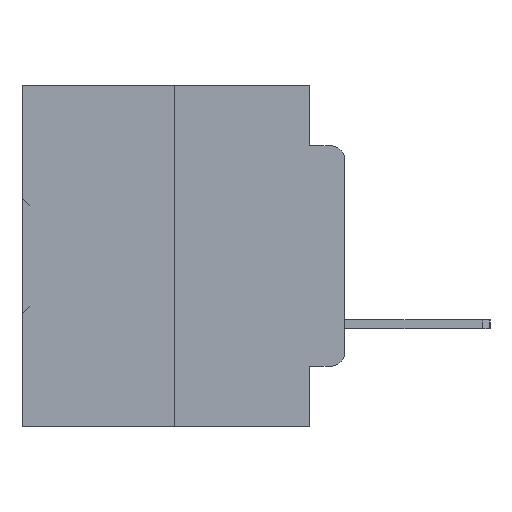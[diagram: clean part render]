
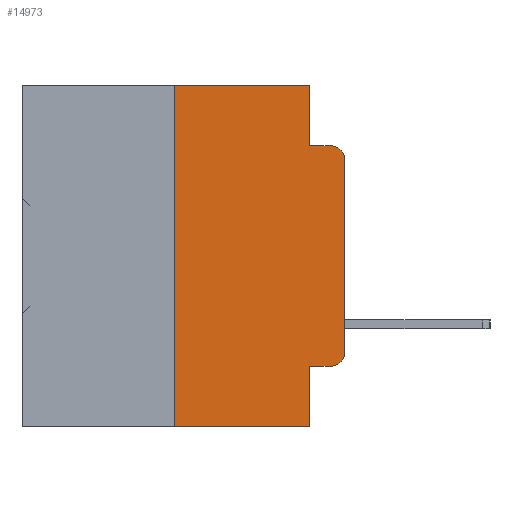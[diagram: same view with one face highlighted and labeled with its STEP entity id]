
A CAD part, left-side view. The second image highlights one B-rep face of the part: STEP entity #14973.
In plain terms, the highlighted planar face has unit normal (-1, 0, 0).
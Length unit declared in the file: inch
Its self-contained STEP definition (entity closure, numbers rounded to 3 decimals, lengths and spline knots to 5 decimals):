
#260 = CARTESIAN_POINT ( 'NONE',  ( 0., 0.25, -0.5 ) ) ;
#705 = VECTOR ( 'NONE', #7834, 39.37008 ) ;
#1303 = EDGE_CURVE ( 'NONE', #7194, #5282, #11119, .T. ) ;
#1907 = CARTESIAN_POINT ( 'NONE',  ( 0., 0.051, -0.4115 ) ) ;
#3157 = ORIENTED_EDGE ( 'NONE', *, *, #1303, .F. ) ;
#3260 = EDGE_CURVE ( 'NONE', #16669, #8296, #23354, .T. ) ;
#4362 = EDGE_CURVE ( 'NONE', #15178, #6514, #33932, .T. ) ;
#4369 = CARTESIAN_POINT ( 'NONE',  ( 0., 0., -0.1085 ) ) ;
#4507 = AXIS2_PLACEMENT_3D ( 'NONE', #18958, #19082, #15504 ) ;
#4655 = LINE ( 'NONE', #19867, #26301 ) ;
#4826 = PLANE ( 'NONE',  #6511 ) ;
#4999 = ORIENTED_EDGE ( 'NONE', *, *, #33340, .T. ) ;
#5282 = VERTEX_POINT ( 'NONE', #15598 ) ;
#5660 = CARTESIAN_POINT ( 'NONE',  ( 0., 0.02, -0.4115 ) ) ;
#5827 = CARTESIAN_POINT ( 'NONE',  ( 0., 0.051, -0.0885 ) ) ;
#5829 = ORIENTED_EDGE ( 'NONE', *, *, #6558, .T. ) ;
#6009 = VECTOR ( 'NONE', #35574, 39.37008 ) ;
#6118 = EDGE_CURVE ( 'NONE', #5282, #16669, #17180, .T. ) ;
#6511 = AXIS2_PLACEMENT_3D ( 'NONE', #24610, #27393, #10530 ) ;
#6514 = VERTEX_POINT ( 'NONE', #28648 ) ;
#6558 = EDGE_CURVE ( 'NONE', #7194, #25589, #17139, .T. ) ;
#7194 = VERTEX_POINT ( 'NONE', #260 ) ;
#7834 = DIRECTION ( 'NONE',  ( 0., 0., -1. ) ) ;
#8296 = VERTEX_POINT ( 'NONE', #5827 ) ;
#8911 = ORIENTED_EDGE ( 'NONE', *, *, #10861, .F. ) ;
#9947 = ORIENTED_EDGE ( 'NONE', *, *, #21044, .F. ) ;
#10082 = DIRECTION ( 'NONE',  ( 0., -1., 0. ) ) ;
#10233 = VECTOR ( 'NONE', #12822, 39.37008 ) ;
#10530 = DIRECTION ( 'NONE',  ( 0., 0., -1. ) ) ;
#10575 = VECTOR ( 'NONE', #10082, 39.37008 ) ;
#10861 = EDGE_CURVE ( 'NONE', #8296, #23716, #4655, .T. ) ;
#11119 = LINE ( 'NONE', #24066, #10233 ) ;
#11692 = DIRECTION ( 'NONE',  ( -1., 0., 0. ) ) ;
#11818 = CARTESIAN_POINT ( 'NONE',  ( 0., 0.02, -0.0885 ) ) ;
#12822 = DIRECTION ( 'NONE',  ( 0., 0., 1. ) ) ;
#14581 = AXIS2_PLACEMENT_3D ( 'NONE', #28563, #11692, #31351 ) ;
#14878 = DIRECTION ( 'NONE',  ( 0., -1., 0. ) ) ;
#14973 = ADVANCED_FACE ( 'NONE', ( #31675 ), #4826, .F. ) ;
#15167 = CARTESIAN_POINT ( 'NONE',  ( 0., 0.051, -0.5 ) ) ;
#15178 = VERTEX_POINT ( 'NONE', #5660 ) ;
#15310 = LINE ( 'NONE', #34096, #29376 ) ;
#15504 = DIRECTION ( 'NONE',  ( 0., 0., -1. ) ) ;
#15598 = CARTESIAN_POINT ( 'NONE',  ( 0., 0.25, 0. ) ) ;
#16669 = VERTEX_POINT ( 'NONE', #34894 ) ;
#16941 = EDGE_LOOP ( 'NONE', ( #32120, #31257, #8911, #18988, #31391, #3157, #5829, #9947, #4999, #34046 ) ) ;
#17139 = LINE ( 'NONE', #31668, #32063 ) ;
#17180 = LINE ( 'NONE', #21353, #10575 ) ;
#17357 = DIRECTION ( 'NONE',  ( 0., 0., 1. ) ) ;
#17743 = VERTEX_POINT ( 'NONE', #4369 ) ;
#18958 = CARTESIAN_POINT ( 'NONE',  ( 0., 0.02, -0.3915 ) ) ;
#18988 = ORIENTED_EDGE ( 'NONE', *, *, #3260, .F. ) ;
#19082 = DIRECTION ( 'NONE',  ( -1., 0., 0. ) ) ;
#19867 = CARTESIAN_POINT ( 'NONE',  ( 0., 0.051, -0.0885 ) ) ;
#21044 = EDGE_CURVE ( 'NONE', #23569, #25589, #23047, .T. ) ;
#21353 = CARTESIAN_POINT ( 'NONE',  ( 0., 0.473, 0. ) ) ;
#21973 = LINE ( 'NONE', #1907, #6009 ) ;
#22466 = CARTESIAN_POINT ( 'NONE',  ( 0., 0.051, -0.4115 ) ) ;
#22725 = DIRECTION ( 'NONE',  ( 0., -1., 0. ) ) ;
#23047 = LINE ( 'NONE', #27847, #29594 ) ;
#23354 = LINE ( 'NONE', #34065, #705 ) ;
#23569 = VERTEX_POINT ( 'NONE', #22466 ) ;
#23716 = VERTEX_POINT ( 'NONE', #11818 ) ;
#24066 = CARTESIAN_POINT ( 'NONE',  ( 0., 0.25, 0. ) ) ;
#24610 = CARTESIAN_POINT ( 'NONE',  ( 0., 0.473, 0. ) ) ;
#25589 = VERTEX_POINT ( 'NONE', #15167 ) ;
#25976 = EDGE_CURVE ( 'NONE', #17743, #23716, #35539, .T. ) ;
#26301 = VECTOR ( 'NONE', #22725, 39.37008 ) ;
#27393 = DIRECTION ( 'NONE',  ( 1., 0., 0. ) ) ;
#27829 = EDGE_CURVE ( 'NONE', #6514, #17743, #15310, .T. ) ;
#27847 = CARTESIAN_POINT ( 'NONE',  ( 0., 0.051, 0. ) ) ;
#28563 = CARTESIAN_POINT ( 'NONE',  ( 0., 0.02, -0.1085 ) ) ;
#28648 = CARTESIAN_POINT ( 'NONE',  ( 0., 0., -0.3915 ) ) ;
#29376 = VECTOR ( 'NONE', #17357, 39.37008 ) ;
#29594 = VECTOR ( 'NONE', #36286, 39.37008 ) ;
#31257 = ORIENTED_EDGE ( 'NONE', *, *, #25976, .T. ) ;
#31351 = DIRECTION ( 'NONE',  ( 0., 0., -1. ) ) ;
#31391 = ORIENTED_EDGE ( 'NONE', *, *, #6118, .F. ) ;
#31668 = CARTESIAN_POINT ( 'NONE',  ( 0., 0.473, -0.5 ) ) ;
#31675 = FACE_OUTER_BOUND ( 'NONE', #16941, .T. ) ;
#32063 = VECTOR ( 'NONE', #14878, 39.37008 ) ;
#32120 = ORIENTED_EDGE ( 'NONE', *, *, #27829, .T. ) ;
#33340 = EDGE_CURVE ( 'NONE', #23569, #15178, #21973, .T. ) ;
#33932 = CIRCLE ( 'NONE', #4507, 0.02 ) ;
#34046 = ORIENTED_EDGE ( 'NONE', *, *, #4362, .T. ) ;
#34065 = CARTESIAN_POINT ( 'NONE',  ( 0., 0.051, 0. ) ) ;
#34096 = CARTESIAN_POINT ( 'NONE',  ( 0., 0., 0. ) ) ;
#34894 = CARTESIAN_POINT ( 'NONE',  ( 0., 0.051, 0. ) ) ;
#35539 = CIRCLE ( 'NONE', #14581, 0.02 ) ;
#35574 = DIRECTION ( 'NONE',  ( 0., -1., 0. ) ) ;
#36286 = DIRECTION ( 'NONE',  ( 0., 0., -1. ) ) ;
